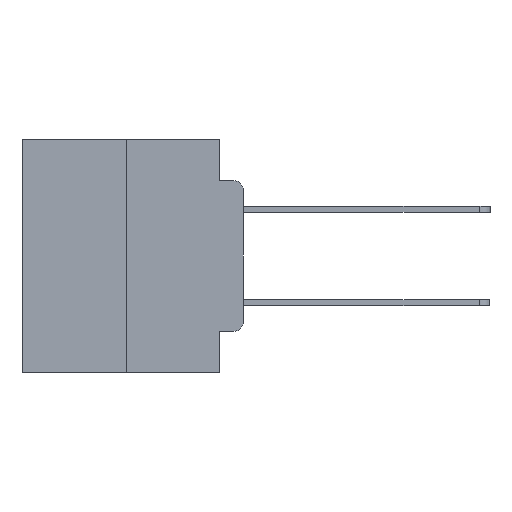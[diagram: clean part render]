
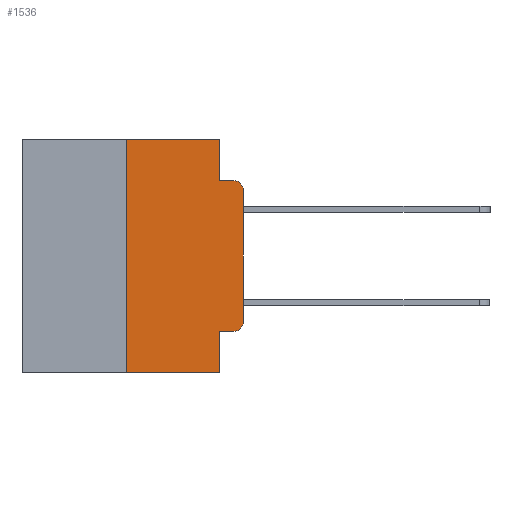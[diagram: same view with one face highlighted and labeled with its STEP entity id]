
A CAD part, left-side view. The second image highlights one B-rep face of the part: STEP entity #1536.
In plain terms, the highlighted planar face has unit normal (-1, 0, 0).
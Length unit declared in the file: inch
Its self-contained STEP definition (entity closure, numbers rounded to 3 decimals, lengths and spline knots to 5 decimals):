
#247 = LINE ( 'NONE', #5257, #19955 ) ;
#256 = ORIENTED_EDGE ( 'NONE', *, *, #22605, .F. ) ;
#774 = CARTESIAN_POINT ( 'NONE',  ( 0., 0.051, 0. ) ) ;
#1265 = ORIENTED_EDGE ( 'NONE', *, *, #2552, .F. ) ;
#1401 = CARTESIAN_POINT ( 'NONE',  ( 0., 0.25, 0. ) ) ;
#1531 = VECTOR ( 'NONE', #3139, 39.37008 ) ;
#1536 = ADVANCED_FACE ( 'NONE', ( #26258 ), #10395, .F. ) ;
#1833 = CIRCLE ( 'NONE', #2737, 0.02 ) ;
#2058 = EDGE_CURVE ( 'NONE', #25069, #3176, #8616, .T. ) ;
#2140 = CARTESIAN_POINT ( 'NONE',  ( 0., 0.02, -0.4115 ) ) ;
#2209 = LINE ( 'NONE', #15089, #1531 ) ;
#2552 = EDGE_CURVE ( 'NONE', #6097, #6544, #2209, .T. ) ;
#2737 = AXIS2_PLACEMENT_3D ( 'NONE', #24235, #24208, #19757 ) ;
#2867 = VERTEX_POINT ( 'NONE', #23677 ) ;
#3139 = DIRECTION ( 'NONE',  ( 0., -1., 0. ) ) ;
#3176 = VERTEX_POINT ( 'NONE', #3627 ) ;
#3462 = CARTESIAN_POINT ( 'NONE',  ( 0., 0.02, -0.3915 ) ) ;
#3504 = VECTOR ( 'NONE', #22286, 39.37008 ) ;
#3619 = VERTEX_POINT ( 'NONE', #22995 ) ;
#3627 = CARTESIAN_POINT ( 'NONE',  ( 0., 0.051, 0. ) ) ;
#3749 = AXIS2_PLACEMENT_3D ( 'NONE', #4214, #17802, #14421 ) ;
#4016 = EDGE_CURVE ( 'NONE', #11357, #6544, #1833, .T. ) ;
#4214 = CARTESIAN_POINT ( 'NONE',  ( 0., 0.473, 0. ) ) ;
#4301 = CARTESIAN_POINT ( 'NONE',  ( 0., 0.25, 0. ) ) ;
#5083 = DIRECTION ( 'NONE',  ( 0., -1., 0. ) ) ;
#5257 = CARTESIAN_POINT ( 'NONE',  ( 0., 0.473, -0.5 ) ) ;
#5603 = DIRECTION ( 'NONE',  ( 0., 0., -1. ) ) ;
#5822 = CARTESIAN_POINT ( 'NONE',  ( 0., 0.051, -0.4115 ) ) ;
#6097 = VERTEX_POINT ( 'NONE', #25975 ) ;
#6544 = VERTEX_POINT ( 'NONE', #11171 ) ;
#7057 = CIRCLE ( 'NONE', #7731, 0.02 ) ;
#7731 = AXIS2_PLACEMENT_3D ( 'NONE', #3462, #18112, #5603 ) ;
#7959 = DIRECTION ( 'NONE',  ( 0., -1., 0. ) ) ;
#8302 = EDGE_CURVE ( 'NONE', #2867, #11357, #20988, .T. ) ;
#8616 = LINE ( 'NONE', #9518, #25603 ) ;
#8672 = ORIENTED_EDGE ( 'NONE', *, *, #18524, .T. ) ;
#9278 = DIRECTION ( 'NONE',  ( 0., -1., 0. ) ) ;
#9328 = DIRECTION ( 'NONE',  ( 0., 0., -1. ) ) ;
#9442 = DIRECTION ( 'NONE',  ( 0., 0., -1. ) ) ;
#9518 = CARTESIAN_POINT ( 'NONE',  ( 0., 0.473, 0. ) ) ;
#9932 = EDGE_CURVE ( 'NONE', #3619, #20906, #247, .T. ) ;
#10021 = CARTESIAN_POINT ( 'NONE',  ( 0., 0., -0.1085 ) ) ;
#10395 = PLANE ( 'NONE',  #3749 ) ;
#10650 = CARTESIAN_POINT ( 'NONE',  ( 0., 0., 0. ) ) ;
#10972 = ORIENTED_EDGE ( 'NONE', *, *, #9932, .T. ) ;
#11171 = CARTESIAN_POINT ( 'NONE',  ( 0., 0.02, -0.0885 ) ) ;
#11357 = VERTEX_POINT ( 'NONE', #10021 ) ;
#12561 = CARTESIAN_POINT ( 'NONE',  ( 0., 0.051, -0.5 ) ) ;
#12602 = VECTOR ( 'NONE', #9328, 39.37008 ) ;
#12665 = VERTEX_POINT ( 'NONE', #18691 ) ;
#13241 = ORIENTED_EDGE ( 'NONE', *, *, #25318, .F. ) ;
#14421 = DIRECTION ( 'NONE',  ( 0., 0., -1. ) ) ;
#15089 = CARTESIAN_POINT ( 'NONE',  ( 0., 0.051, -0.0885 ) ) ;
#15205 = ORIENTED_EDGE ( 'NONE', *, *, #2058, .F. ) ;
#15525 = ORIENTED_EDGE ( 'NONE', *, *, #17170, .T. ) ;
#16083 = VECTOR ( 'NONE', #9442, 39.37008 ) ;
#16456 = ORIENTED_EDGE ( 'NONE', *, *, #23969, .F. ) ;
#16776 = ORIENTED_EDGE ( 'NONE', *, *, #8302, .T. ) ;
#17170 = EDGE_CURVE ( 'NONE', #20978, #2867, #7057, .T. ) ;
#17802 = DIRECTION ( 'NONE',  ( 1., 0., 0. ) ) ;
#18046 = ORIENTED_EDGE ( 'NONE', *, *, #4016, .T. ) ;
#18052 = LINE ( 'NONE', #774, #12602 ) ;
#18112 = DIRECTION ( 'NONE',  ( -1., 0., 0. ) ) ;
#18524 = EDGE_CURVE ( 'NONE', #12665, #20978, #22151, .T. ) ;
#18691 = CARTESIAN_POINT ( 'NONE',  ( 0., 0.051, -0.4115 ) ) ;
#19757 = DIRECTION ( 'NONE',  ( 0., 0., -1. ) ) ;
#19955 = VECTOR ( 'NONE', #5083, 39.37008 ) ;
#20351 = VECTOR ( 'NONE', #22879, 39.37008 ) ;
#20906 = VERTEX_POINT ( 'NONE', #12561 ) ;
#20978 = VERTEX_POINT ( 'NONE', #2140 ) ;
#20988 = LINE ( 'NONE', #10650, #20351 ) ;
#21534 = VECTOR ( 'NONE', #7959, 39.37008 ) ;
#22106 = LINE ( 'NONE', #23774, #16083 ) ;
#22151 = LINE ( 'NONE', #5822, #21534 ) ;
#22286 = DIRECTION ( 'NONE',  ( 0., 0., 1. ) ) ;
#22605 = EDGE_CURVE ( 'NONE', #12665, #20906, #22106, .T. ) ;
#22879 = DIRECTION ( 'NONE',  ( 0., 0., 1. ) ) ;
#22995 = CARTESIAN_POINT ( 'NONE',  ( 0., 0.25, -0.5 ) ) ;
#23677 = CARTESIAN_POINT ( 'NONE',  ( 0., 0., -0.3915 ) ) ;
#23774 = CARTESIAN_POINT ( 'NONE',  ( 0., 0.051, 0. ) ) ;
#23969 = EDGE_CURVE ( 'NONE', #3619, #25069, #25516, .T. ) ;
#24208 = DIRECTION ( 'NONE',  ( -1., 0., 0. ) ) ;
#24235 = CARTESIAN_POINT ( 'NONE',  ( 0., 0.02, -0.1085 ) ) ;
#25069 = VERTEX_POINT ( 'NONE', #4301 ) ;
#25318 = EDGE_CURVE ( 'NONE', #3176, #6097, #18052, .T. ) ;
#25409 = EDGE_LOOP ( 'NONE', ( #16776, #18046, #1265, #13241, #15205, #16456, #10972, #256, #8672, #15525 ) ) ;
#25516 = LINE ( 'NONE', #1401, #3504 ) ;
#25603 = VECTOR ( 'NONE', #9278, 39.37008 ) ;
#25975 = CARTESIAN_POINT ( 'NONE',  ( 0., 0.051, -0.0885 ) ) ;
#26258 = FACE_OUTER_BOUND ( 'NONE', #25409, .T. ) ;
